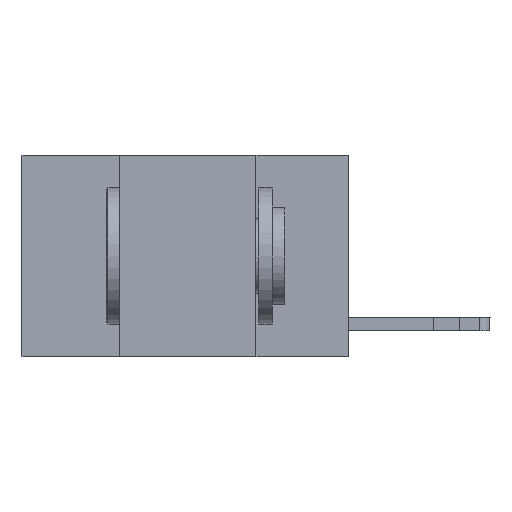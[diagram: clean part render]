
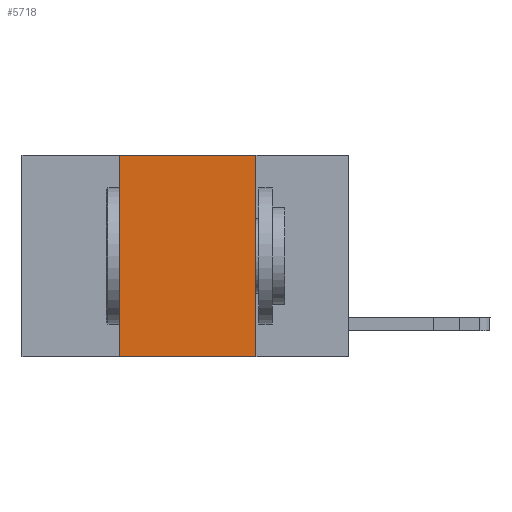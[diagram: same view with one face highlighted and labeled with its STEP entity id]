
A CAD part, left-side view. The second image highlights one B-rep face of the part: STEP entity #5718.
In plain terms, the highlighted planar face has unit normal (-1, 0, 0).
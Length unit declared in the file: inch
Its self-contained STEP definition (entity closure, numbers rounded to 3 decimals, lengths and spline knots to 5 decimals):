
#205 = CARTESIAN_POINT ( 'NONE',  ( 0., 0.17, -0.37 ) ) ;
#233 = DIRECTION ( 'NONE',  ( 0., -1., 0. ) ) ;
#779 = EDGE_CURVE ( 'NONE', #5334, #4093, #2214, .T. ) ;
#1904 = VECTOR ( 'NONE', #233, 39.37008 ) ;
#2214 = LINE ( 'NONE', #8635, #1904 ) ;
#2247 = ORIENTED_EDGE ( 'NONE', *, *, #13735, .F. ) ;
#2676 = ORIENTED_EDGE ( 'NONE', *, *, #3388, .T. ) ;
#2686 = AXIS2_PLACEMENT_3D ( 'NONE', #3125, #7473, #13105 ) ;
#2816 = VECTOR ( 'NONE', #3535, 39.37008 ) ;
#3125 = CARTESIAN_POINT ( 'NONE',  ( 0., 0.6, 0. ) ) ;
#3388 = EDGE_CURVE ( 'NONE', #8409, #9860, #12367, .T. ) ;
#3535 = DIRECTION ( 'NONE',  ( 0., -1., 0. ) ) ;
#3830 = CARTESIAN_POINT ( 'NONE',  ( 0., 0.42, 0. ) ) ;
#3884 = CARTESIAN_POINT ( 'NONE',  ( 0., 0.17, 0. ) ) ;
#4093 = VERTEX_POINT ( 'NONE', #8629 ) ;
#4438 = CARTESIAN_POINT ( 'NONE',  ( 0., 0.42, 0. ) ) ;
#4578 = ORIENTED_EDGE ( 'NONE', *, *, #779, .F. ) ;
#5334 = VERTEX_POINT ( 'NONE', #4438 ) ;
#5718 = ADVANCED_FACE ( 'NONE', ( #12891 ), #8691, .F. ) ;
#6625 = LINE ( 'NONE', #3830, #8929 ) ;
#7473 = DIRECTION ( 'NONE',  ( 1., 0., 0. ) ) ;
#8184 = CARTESIAN_POINT ( 'NONE',  ( 0., 0.42, -0.37 ) ) ;
#8215 = DIRECTION ( 'NONE',  ( 0., 0., -1. ) ) ;
#8409 = VERTEX_POINT ( 'NONE', #8184 ) ;
#8629 = CARTESIAN_POINT ( 'NONE',  ( 0., 0.17, 0. ) ) ;
#8635 = CARTESIAN_POINT ( 'NONE',  ( 0., 0.6, 0. ) ) ;
#8691 = PLANE ( 'NONE',  #2686 ) ;
#8929 = VECTOR ( 'NONE', #11121, 39.37008 ) ;
#9860 = VERTEX_POINT ( 'NONE', #205 ) ;
#10173 = CARTESIAN_POINT ( 'NONE',  ( 0., 0.6, -0.37 ) ) ;
#10316 = LINE ( 'NONE', #3884, #11900 ) ;
#11121 = DIRECTION ( 'NONE',  ( 0., 0., 1. ) ) ;
#11461 = EDGE_LOOP ( 'NONE', ( #2247, #4578, #12817, #2676 ) ) ;
#11900 = VECTOR ( 'NONE', #8215, 39.37008 ) ;
#12367 = LINE ( 'NONE', #10173, #2816 ) ;
#12817 = ORIENTED_EDGE ( 'NONE', *, *, #13329, .F. ) ;
#12891 = FACE_OUTER_BOUND ( 'NONE', #11461, .T. ) ;
#13105 = DIRECTION ( 'NONE',  ( 0., 0., -1. ) ) ;
#13329 = EDGE_CURVE ( 'NONE', #8409, #5334, #6625, .T. ) ;
#13735 = EDGE_CURVE ( 'NONE', #4093, #9860, #10316, .T. ) ;
